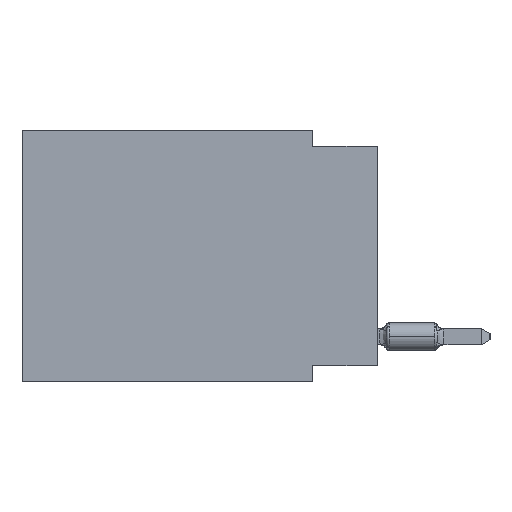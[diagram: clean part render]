
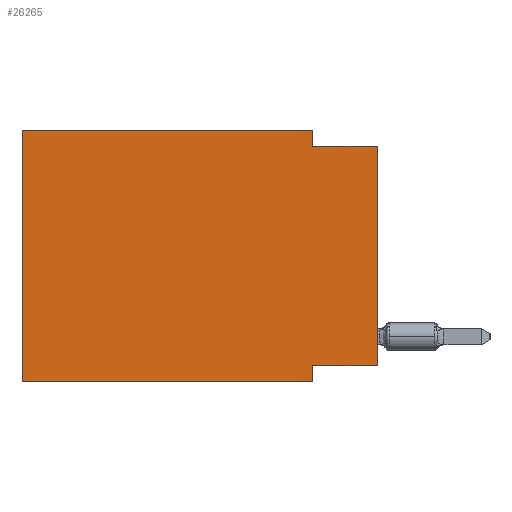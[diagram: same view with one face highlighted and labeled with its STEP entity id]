
A CAD part, left-side view. The second image highlights one B-rep face of the part: STEP entity #26265.
In plain terms, the highlighted planar face has unit normal (-1, 0, 0).
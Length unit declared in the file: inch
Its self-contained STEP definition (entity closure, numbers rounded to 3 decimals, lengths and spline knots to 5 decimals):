
#1223 = DIRECTION ( 'NONE',  ( 0., -1., 0. ) ) ;
#1245 = VERTEX_POINT ( 'NONE', #5341 ) ;
#1503 = LINE ( 'NONE', #24160, #9858 ) ;
#1631 = LINE ( 'NONE', #7657, #4411 ) ;
#2056 = EDGE_CURVE ( 'NONE', #11666, #2533, #11919, .T. ) ;
#2286 = VECTOR ( 'NONE', #1223, 39.37008 ) ;
#2533 = VERTEX_POINT ( 'NONE', #4714 ) ;
#2768 = LINE ( 'NONE', #23665, #22761 ) ;
#3257 = VERTEX_POINT ( 'NONE', #6894 ) ;
#3883 = VECTOR ( 'NONE', #13665, 39.37008 ) ;
#4041 = AXIS2_PLACEMENT_3D ( 'NONE', #8842, #15155, #16618 ) ;
#4159 = DIRECTION ( 'NONE',  ( 0., 0., 1. ) ) ;
#4287 = CARTESIAN_POINT ( 'NONE',  ( 0., 0.55, 0. ) ) ;
#4411 = VECTOR ( 'NONE', #22404, 39.37008 ) ;
#4696 = VECTOR ( 'NONE', #6601, 39.37008 ) ;
#4714 = CARTESIAN_POINT ( 'NONE',  ( 0., 0.55, 0. ) ) ;
#5341 = CARTESIAN_POINT ( 'NONE',  ( 0., 0.1, 0. ) ) ;
#5802 = DIRECTION ( 'NONE',  ( 0., 0., -1. ) ) ;
#5910 = CARTESIAN_POINT ( 'NONE',  ( 0., 0.55, -0.39 ) ) ;
#6065 = FACE_OUTER_BOUND ( 'NONE', #6839, .T. ) ;
#6601 = DIRECTION ( 'NONE',  ( 0., 1., 0. ) ) ;
#6771 = ORIENTED_EDGE ( 'NONE', *, *, #17608, .F. ) ;
#6839 = EDGE_LOOP ( 'NONE', ( #18529, #6771, #9937, #17962, #21642, #24134, #21121, #18871 ) ) ;
#6894 = CARTESIAN_POINT ( 'NONE',  ( 0., 0., -0.365 ) ) ;
#7050 = CARTESIAN_POINT ( 'NONE',  ( 0., 0.1, -0.39 ) ) ;
#7095 = EDGE_CURVE ( 'NONE', #2533, #1245, #7123, .T. ) ;
#7123 = LINE ( 'NONE', #21594, #22280 ) ;
#7657 = CARTESIAN_POINT ( 'NONE',  ( 0., 0., -0.025 ) ) ;
#8229 = CARTESIAN_POINT ( 'NONE',  ( 0., 0.1, -0.365 ) ) ;
#8842 = CARTESIAN_POINT ( 'NONE',  ( 0., 0.55, 0. ) ) ;
#9519 = LINE ( 'NONE', #10036, #3883 ) ;
#9749 = LINE ( 'NONE', #5910, #2286 ) ;
#9858 = VECTOR ( 'NONE', #5802, 39.37008 ) ;
#9937 = ORIENTED_EDGE ( 'NONE', *, *, #15296, .F. ) ;
#9952 = EDGE_CURVE ( 'NONE', #3257, #14171, #2768, .T. ) ;
#10036 = CARTESIAN_POINT ( 'NONE',  ( 0., 0.1, -0.39 ) ) ;
#11040 = DIRECTION ( 'NONE',  ( 0., 0., 1. ) ) ;
#11362 = VERTEX_POINT ( 'NONE', #8229 ) ;
#11666 = VERTEX_POINT ( 'NONE', #16107 ) ;
#11848 = EDGE_CURVE ( 'NONE', #3257, #11362, #16769, .T. ) ;
#11919 = LINE ( 'NONE', #4287, #12363 ) ;
#12363 = VECTOR ( 'NONE', #4159, 39.37008 ) ;
#13665 = DIRECTION ( 'NONE',  ( 0., 0., -1. ) ) ;
#14171 = VERTEX_POINT ( 'NONE', #17108 ) ;
#14471 = CARTESIAN_POINT ( 'NONE',  ( 0., 0., -0.365 ) ) ;
#15155 = DIRECTION ( 'NONE',  ( 1., 0., 0. ) ) ;
#15268 = EDGE_CURVE ( 'NONE', #11362, #25125, #9519, .T. ) ;
#15296 = EDGE_CURVE ( 'NONE', #1245, #26078, #1503, .T. ) ;
#16107 = CARTESIAN_POINT ( 'NONE',  ( 0., 0.55, -0.39 ) ) ;
#16618 = DIRECTION ( 'NONE',  ( 0., 0., -1. ) ) ;
#16769 = LINE ( 'NONE', #14471, #4696 ) ;
#16894 = PLANE ( 'NONE',  #4041 ) ;
#17108 = CARTESIAN_POINT ( 'NONE',  ( 0., 0., -0.025 ) ) ;
#17608 = EDGE_CURVE ( 'NONE', #26078, #14171, #1631, .T. ) ;
#17962 = ORIENTED_EDGE ( 'NONE', *, *, #7095, .F. ) ;
#18529 = ORIENTED_EDGE ( 'NONE', *, *, #9952, .T. ) ;
#18871 = ORIENTED_EDGE ( 'NONE', *, *, #11848, .F. ) ;
#21121 = ORIENTED_EDGE ( 'NONE', *, *, #15268, .F. ) ;
#21594 = CARTESIAN_POINT ( 'NONE',  ( 0., 0.55, 0. ) ) ;
#21642 = ORIENTED_EDGE ( 'NONE', *, *, #2056, .F. ) ;
#22280 = VECTOR ( 'NONE', #25726, 39.37008 ) ;
#22404 = DIRECTION ( 'NONE',  ( 0., -1., 0. ) ) ;
#22761 = VECTOR ( 'NONE', #11040, 39.37008 ) ;
#22911 = EDGE_CURVE ( 'NONE', #11666, #25125, #9749, .T. ) ;
#23665 = CARTESIAN_POINT ( 'NONE',  ( 0., 0., 0. ) ) ;
#23885 = CARTESIAN_POINT ( 'NONE',  ( 0., 0.1, -0.025 ) ) ;
#24134 = ORIENTED_EDGE ( 'NONE', *, *, #22911, .T. ) ;
#24160 = CARTESIAN_POINT ( 'NONE',  ( 0., 0.1, 0. ) ) ;
#25125 = VERTEX_POINT ( 'NONE', #7050 ) ;
#25726 = DIRECTION ( 'NONE',  ( 0., -1., 0. ) ) ;
#26078 = VERTEX_POINT ( 'NONE', #23885 ) ;
#26265 = ADVANCED_FACE ( 'NONE', ( #6065 ), #16894, .F. ) ;
